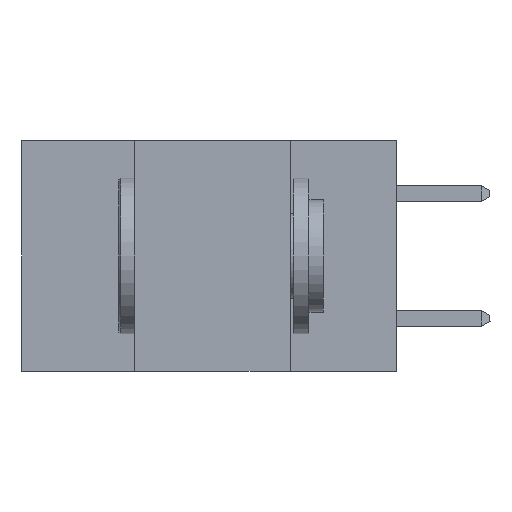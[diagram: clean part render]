
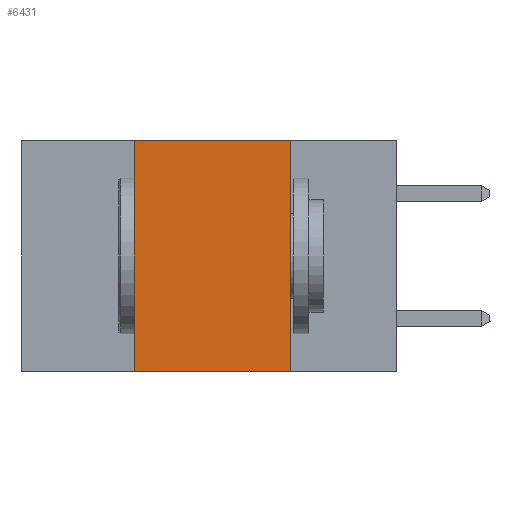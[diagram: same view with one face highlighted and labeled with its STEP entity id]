
A CAD part, left-side view. The second image highlights one B-rep face of the part: STEP entity #6431.
In plain terms, the highlighted planar face has unit normal (-1, 0, 0).
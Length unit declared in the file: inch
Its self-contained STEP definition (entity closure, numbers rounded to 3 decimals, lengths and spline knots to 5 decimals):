
#345 = CARTESIAN_POINT ( 'NONE',  ( 0., 0.6, 0. ) ) ;
#364 = VERTEX_POINT ( 'NONE', #5703 ) ;
#992 = CARTESIAN_POINT ( 'NONE',  ( 0., 0.6, 0. ) ) ;
#1024 = DIRECTION ( 'NONE',  ( 0., -1., 0. ) ) ;
#1325 = LINE ( 'NONE', #9374, #3168 ) ;
#1374 = CARTESIAN_POINT ( 'NONE',  ( 0., 0.17, -0.37 ) ) ;
#2478 = LINE ( 'NONE', #992, #3817 ) ;
#2685 = DIRECTION ( 'NONE',  ( 1., 0., 0. ) ) ;
#3168 = VECTOR ( 'NONE', #8513, 39.37008 ) ;
#3288 = EDGE_CURVE ( 'NONE', #9463, #364, #2478, .T. ) ;
#3422 = EDGE_CURVE ( 'NONE', #6825, #9463, #9598, .T. ) ;
#3817 = VECTOR ( 'NONE', #1024, 39.37008 ) ;
#4054 = EDGE_CURVE ( 'NONE', #6825, #8808, #1325, .T. ) ;
#4516 = ORIENTED_EDGE ( 'NONE', *, *, #8033, .F. ) ;
#4631 = CARTESIAN_POINT ( 'NONE',  ( 0., 0.42, 0. ) ) ;
#4730 = PLANE ( 'NONE',  #7676 ) ;
#5148 = CARTESIAN_POINT ( 'NONE',  ( 0., 0.17, 0. ) ) ;
#5703 = CARTESIAN_POINT ( 'NONE',  ( 0., 0.17, 0. ) ) ;
#6431 = ADVANCED_FACE ( 'NONE', ( #9735 ), #4730, .F. ) ;
#6524 = LINE ( 'NONE', #5148, #8477 ) ;
#6650 = VECTOR ( 'NONE', #10015, 39.37008 ) ;
#6825 = VERTEX_POINT ( 'NONE', #8175 ) ;
#7018 = ORIENTED_EDGE ( 'NONE', *, *, #4054, .T. ) ;
#7242 = DIRECTION ( 'NONE',  ( 0., 0., -1. ) ) ;
#7278 = EDGE_LOOP ( 'NONE', ( #4516, #8733, #8440, #7018 ) ) ;
#7676 = AXIS2_PLACEMENT_3D ( 'NONE', #345, #2685, #7242 ) ;
#8033 = EDGE_CURVE ( 'NONE', #364, #8808, #6524, .T. ) ;
#8175 = CARTESIAN_POINT ( 'NONE',  ( 0., 0.42, -0.37 ) ) ;
#8178 = DIRECTION ( 'NONE',  ( 0., 0., -1. ) ) ;
#8440 = ORIENTED_EDGE ( 'NONE', *, *, #3422, .F. ) ;
#8477 = VECTOR ( 'NONE', #8178, 39.37008 ) ;
#8513 = DIRECTION ( 'NONE',  ( 0., -1., 0. ) ) ;
#8733 = ORIENTED_EDGE ( 'NONE', *, *, #3288, .F. ) ;
#8808 = VERTEX_POINT ( 'NONE', #1374 ) ;
#9105 = CARTESIAN_POINT ( 'NONE',  ( 0., 0.42, 0. ) ) ;
#9374 = CARTESIAN_POINT ( 'NONE',  ( 0., 0.6, -0.37 ) ) ;
#9463 = VERTEX_POINT ( 'NONE', #4631 ) ;
#9598 = LINE ( 'NONE', #9105, #6650 ) ;
#9735 = FACE_OUTER_BOUND ( 'NONE', #7278, .T. ) ;
#10015 = DIRECTION ( 'NONE',  ( 0., 0., 1. ) ) ;
